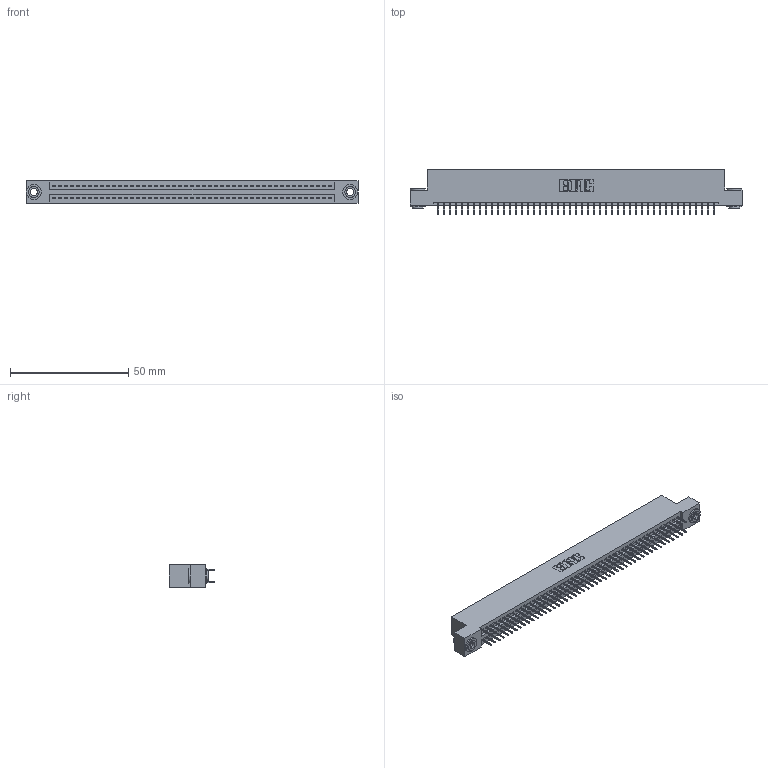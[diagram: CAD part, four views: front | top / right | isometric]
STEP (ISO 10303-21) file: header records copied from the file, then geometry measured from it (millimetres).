
FILE_DESCRIPTION (( 'STEP AP203' ), '1' );
FILE_NAME ('345-094-524-203.STEP', '2018-10-05T00:10:35', ( '' ), ( '' ), 'SwSTEP 2.0', 'SolidWorks 2016', '' );
FILE_SCHEMA (( 'CONFIG_CONTROL_DESIGN' ));
Length unit declared in the file: inch
Products named in the file (4): 345-094-524-203; 345-292-001_345-293-124; 345 Part_Flush Mounting Lugs - 0.156 Dia-TH; 345-250-002_345-250-002-102
Assembly tree (97 placements, depth 2):
  345-094-524-203
    345 Part_Flush Mounting Lugs - 0.156 Dia-TH
    345-292-001_345-293-124  x94
    345-250-002_345-250-002-102  x2
Bounding box: 140.59 x 19.35 x 9.4 mm (x, y, z)
Volume: 13580.5 mm3; surface area: 20000.5 mm2
Topology: 97 solids, 97 shells, 5240 faces, 14799 edges, 9486 vertices
Faces by surface type: plane 3756, cylinder 1476, cone 8
Entity records: 36928 total; most frequent: CARTESIAN_POINT 6159, ORIENTED_EDGE 6086, DIRECTION 5457, EDGE_CURVE 3043, LINE 2703, VECTOR 2703, VERTEX_POINT 2022, AXIS2_PLACEMENT_3D 1377
